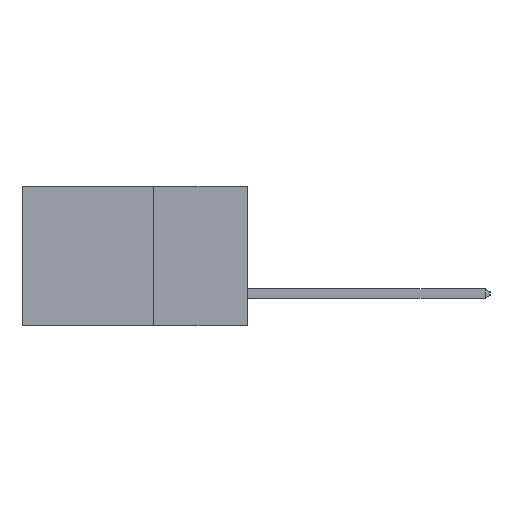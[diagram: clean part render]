
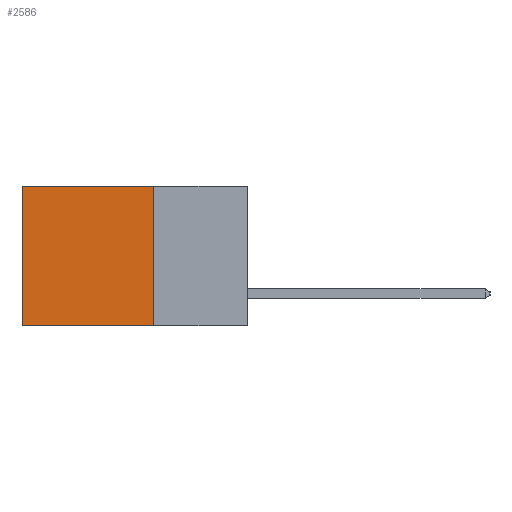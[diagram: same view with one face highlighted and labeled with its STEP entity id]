
A CAD part, left-side view. The second image highlights one B-rep face of the part: STEP entity #2586.
In plain terms, the highlighted planar face has unit normal (-1, 0, 0).
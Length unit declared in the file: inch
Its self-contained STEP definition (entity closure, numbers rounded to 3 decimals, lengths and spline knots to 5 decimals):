
#1603 = CARTESIAN_POINT ( 'NONE',  ( 0.298, 0.25, 0. ) ) ;
#1726 = EDGE_CURVE ( 'NONE', #4264, #6295, #18766, .T. ) ;
#2248 = PLANE ( 'NONE',  #6975 ) ;
#2413 = CARTESIAN_POINT ( 'NONE',  ( 0.298, 0.25, -0.37 ) ) ;
#2586 = ADVANCED_FACE ( 'NONE', ( #11532 ), #2248, .F. ) ;
#3099 = VECTOR ( 'NONE', #18499, 39.37008 ) ;
#4264 = VERTEX_POINT ( 'NONE', #15467 ) ;
#5679 = VECTOR ( 'NONE', #5745, 39.37008 ) ;
#5745 = DIRECTION ( 'NONE',  ( 0., 0., -1. ) ) ;
#5861 = ORIENTED_EDGE ( 'NONE', *, *, #13852, .T. ) ;
#6295 = VERTEX_POINT ( 'NONE', #2413 ) ;
#6831 = CARTESIAN_POINT ( 'NONE',  ( 0.298, 0.25, -0.37 ) ) ;
#6975 = AXIS2_PLACEMENT_3D ( 'NONE', #1603, #8947, #8992 ) ;
#6978 = VECTOR ( 'NONE', #8097, 39.37008 ) ;
#7100 = DIRECTION ( 'NONE',  ( 0., 0., -1. ) ) ;
#7157 = VECTOR ( 'NONE', #7100, 39.37008 ) ;
#8097 = DIRECTION ( 'NONE',  ( 0., 1., 0. ) ) ;
#8947 = DIRECTION ( 'NONE',  ( 1., 0., 0. ) ) ;
#8992 = DIRECTION ( 'NONE',  ( 0., 0., -1. ) ) ;
#9763 = ORIENTED_EDGE ( 'NONE', *, *, #11783, .T. ) ;
#11532 = FACE_OUTER_BOUND ( 'NONE', #15001, .T. ) ;
#11783 = EDGE_CURVE ( 'NONE', #15701, #18834, #13542, .T. ) ;
#13094 = ORIENTED_EDGE ( 'NONE', *, *, #1726, .F. ) ;
#13542 = LINE ( 'NONE', #18843, #5679 ) ;
#13852 = EDGE_CURVE ( 'NONE', #4264, #15701, #18156, .T. ) ;
#14968 = CARTESIAN_POINT ( 'NONE',  ( 0.298, 0.25, 0. ) ) ;
#15001 = EDGE_LOOP ( 'NONE', ( #9763, #17487, #13094, #5861 ) ) ;
#15467 = CARTESIAN_POINT ( 'NONE',  ( 0.298, 0.25, 0. ) ) ;
#15701 = VERTEX_POINT ( 'NONE', #17359 ) ;
#16351 = CARTESIAN_POINT ( 'NONE',  ( 0.298, 0.6, -0.37 ) ) ;
#16842 = CARTESIAN_POINT ( 'NONE',  ( 0.298, 0.25, 0. ) ) ;
#17359 = CARTESIAN_POINT ( 'NONE',  ( 0.298, 0.6, 0. ) ) ;
#17487 = ORIENTED_EDGE ( 'NONE', *, *, #18519, .F. ) ;
#17728 = LINE ( 'NONE', #6831, #3099 ) ;
#18156 = LINE ( 'NONE', #16842, #6978 ) ;
#18499 = DIRECTION ( 'NONE',  ( 0., 1., 0. ) ) ;
#18519 = EDGE_CURVE ( 'NONE', #6295, #18834, #17728, .T. ) ;
#18766 = LINE ( 'NONE', #14968, #7157 ) ;
#18834 = VERTEX_POINT ( 'NONE', #16351 ) ;
#18843 = CARTESIAN_POINT ( 'NONE',  ( 0.298, 0.6, 0. ) ) ;
